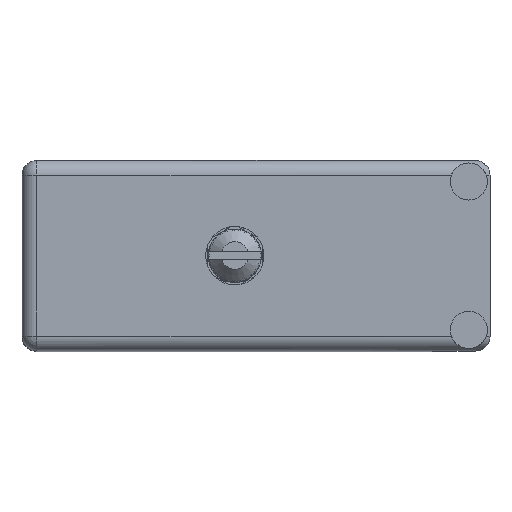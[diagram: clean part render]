
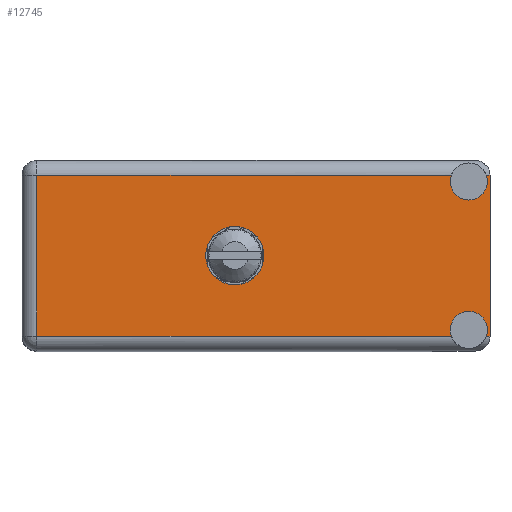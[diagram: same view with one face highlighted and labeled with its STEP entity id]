
A CAD part, top view. The second image highlights one B-rep face of the part: STEP entity #12745.
In plain terms, the highlighted face is planar.
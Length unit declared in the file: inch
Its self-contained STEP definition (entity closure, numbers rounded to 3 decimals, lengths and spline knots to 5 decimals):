
#2591 = CARTESIAN_POINT ( 'NONE',  ( 1.004, 1.566, -0.587 ) ) ;
#3348 = CARTESIAN_POINT ( 'NONE',  ( 2.208, 1.566, 0. ) ) ;
#3877 = DIRECTION ( 'NONE',  ( 0., 0., 1. ) ) ;
#5024 = ORIENTED_EDGE ( 'NONE', *, *, #66729, .F. ) ;
#6600 = EDGE_CURVE ( 'NONE', #48146, #54085, #84468, .T. ) ;
#7967 = CIRCLE ( 'NONE', #73223, 0.1375 ) ;
#8674 = VERTEX_POINT ( 'NONE', #111111 ) ;
#8995 = ORIENTED_EDGE ( 'NONE', *, *, #95544, .F. ) ;
#9302 = DIRECTION ( 'NONE',  ( 0., 1., 0. ) ) ;
#10871 = EDGE_CURVE ( 'NONE', #8674, #36048, #101424, .T. ) ;
#10915 = DIRECTION ( 'NONE',  ( 0., 1., 0. ) ) ;
#11026 = DIRECTION ( 'NONE',  ( 0., 0., 1. ) ) ;
#12745 = ADVANCED_FACE ( 'NONE', ( #70120, #63088 ), #25785, .T. ) ;
#13335 = CARTESIAN_POINT ( 'NONE',  ( 2.108, 1.566, -0.0995 ) ) ;
#14721 = CARTESIAN_POINT ( 'NONE',  ( 2.19038, 1.566, -0.829 ) ) ;
#14968 = VERTEX_POINT ( 'NONE', #64143 ) ;
#16832 = CARTESIAN_POINT ( 'NONE',  ( 2.208, 1.566, -0.07 ) ) ;
#19251 = AXIS2_PLACEMENT_3D ( 'NONE', #72174, #19673, #55251 ) ;
#19673 = DIRECTION ( 'NONE',  ( 0., 1., 0. ) ) ;
#19711 = CARTESIAN_POINT ( 'NONE',  ( 2.108, 1.566, -0.7995 ) ) ;
#20276 = ORIENTED_EDGE ( 'NONE', *, *, #80384, .F. ) ;
#20777 = CARTESIAN_POINT ( 'NONE',  ( 1.004, 1.566, -0.312 ) ) ;
#23795 = DIRECTION ( 'NONE',  ( 0., 1., 0. ) ) ;
#25191 = LINE ( 'NONE', #61328, #69030 ) ;
#25785 = PLANE ( 'NONE',  #48357 ) ;
#28217 = DIRECTION ( 'NONE',  ( 1., 0., 0. ) ) ;
#28290 = EDGE_CURVE ( 'NONE', #70112, #35660, #99480, .T. ) ;
#29414 = DIRECTION ( 'NONE',  ( -1., 0., 0. ) ) ;
#29983 = ORIENTED_EDGE ( 'NONE', *, *, #45048, .F. ) ;
#30731 = ORIENTED_EDGE ( 'NONE', *, *, #94817, .T. ) ;
#31386 = AXIS2_PLACEMENT_3D ( 'NONE', #69862, #23795, #96119 ) ;
#32620 = CARTESIAN_POINT ( 'NONE',  ( 2.208, 1.566, -0.07 ) ) ;
#32815 = EDGE_CURVE ( 'NONE', #98189, #36048, #72546, .T. ) ;
#33254 = DIRECTION ( 'NONE',  ( 0., 1., 0. ) ) ;
#35660 = VERTEX_POINT ( 'NONE', #14721 ) ;
#36048 = VERTEX_POINT ( 'NONE', #16832 ) ;
#37917 = EDGE_LOOP ( 'NONE', ( #64680, #20276, #29983, #110406, #106942, #49056, #84416, #5024, #30731, #51431 ) ) ;
#44961 = EDGE_LOOP ( 'NONE', ( #107424, #8995 ) ) ;
#45048 = EDGE_CURVE ( 'NONE', #98189, #50715, #107716, .T. ) ;
#45670 = LINE ( 'NONE', #81244, #69245 ) ;
#48146 = VERTEX_POINT ( 'NONE', #20777 ) ;
#48357 = AXIS2_PLACEMENT_3D ( 'NONE', #88787, #69545, #98694 ) ;
#48472 = CARTESIAN_POINT ( 'NONE',  ( 0.07, 1.566, -0.829 ) ) ;
#48623 = AXIS2_PLACEMENT_3D ( 'NONE', #19711, #10915, #3877 ) ;
#49056 = ORIENTED_EDGE ( 'NONE', *, *, #90664, .T. ) ;
#50715 = VERTEX_POINT ( 'NONE', #60474 ) ;
#51148 = EDGE_CURVE ( 'NONE', #55655, #14968, #25191, .T. ) ;
#51431 = ORIENTED_EDGE ( 'NONE', *, *, #51148, .T. ) ;
#53678 = CARTESIAN_POINT ( 'NONE',  ( 1.004, 1.566, -0.4495 ) ) ;
#53772 = CIRCLE ( 'NONE', #31386, 0.0875 ) ;
#54085 = VERTEX_POINT ( 'NONE', #2591 ) ;
#54191 = CIRCLE ( 'NONE', #48623, 0.0875 ) ;
#55251 = DIRECTION ( 'NONE',  ( 0., 0., 1. ) ) ;
#55655 = VERTEX_POINT ( 'NONE', #48472 ) ;
#60474 = CARTESIAN_POINT ( 'NONE',  ( 2.108, 1.566, -0.187 ) ) ;
#60769 = DIRECTION ( 'NONE',  ( 0., 0., 1. ) ) ;
#61328 = CARTESIAN_POINT ( 'NONE',  ( 0.07, 1.566, -0.899 ) ) ;
#63088 = FACE_OUTER_BOUND ( 'NONE', #37917, .T. ) ;
#64143 = CARTESIAN_POINT ( 'NONE',  ( 0.07, 1.566, -0.07 ) ) ;
#64680 = ORIENTED_EDGE ( 'NONE', *, *, #108766, .T. ) ;
#66729 = EDGE_CURVE ( 'NONE', #109293, #70112, #54191, .T. ) ;
#67032 = LINE ( 'NONE', #32620, #83664 ) ;
#67667 = CARTESIAN_POINT ( 'NONE',  ( 2.108, 1.566, -0.7995 ) ) ;
#69030 = VECTOR ( 'NONE', #60769, 39.37008 ) ;
#69245 = VECTOR ( 'NONE', #72466, 39.37008 ) ;
#69545 = DIRECTION ( 'NONE',  ( 0., 1., 0. ) ) ;
#69606 = CARTESIAN_POINT ( 'NONE',  ( 2.108, 1.566, -0.712 ) ) ;
#69862 = CARTESIAN_POINT ( 'NONE',  ( 2.108, 1.566, -0.0995 ) ) ;
#70112 = VERTEX_POINT ( 'NONE', #69606 ) ;
#70120 = FACE_BOUND ( 'NONE', #44961, .T. ) ;
#72174 = CARTESIAN_POINT ( 'NONE',  ( 1.004, 1.566, -0.4495 ) ) ;
#72403 = VECTOR ( 'NONE', #100266, 39.37008 ) ;
#72466 = DIRECTION ( 'NONE',  ( -1., 0., 0. ) ) ;
#72546 = LINE ( 'NONE', #74698, #106995 ) ;
#72921 = VERTEX_POINT ( 'NONE', #98402 ) ;
#73223 = AXIS2_PLACEMENT_3D ( 'NONE', #53678, #9302, #11026 ) ;
#74698 = CARTESIAN_POINT ( 'NONE',  ( 2.208, 1.566, -0.07 ) ) ;
#75477 = CARTESIAN_POINT ( 'NONE',  ( 0., 1.566, -0.829 ) ) ;
#76357 = DIRECTION ( 'NONE',  ( 1., 0., 0. ) ) ;
#78912 = VECTOR ( 'NONE', #29414, 39.37008 ) ;
#80384 = EDGE_CURVE ( 'NONE', #50715, #72921, #53772, .T. ) ;
#81244 = CARTESIAN_POINT ( 'NONE',  ( 0., 1.566, -0.829 ) ) ;
#82643 = AXIS2_PLACEMENT_3D ( 'NONE', #67667, #33254, #94508 ) ;
#83664 = VECTOR ( 'NONE', #76357, 39.37008 ) ;
#84416 = ORIENTED_EDGE ( 'NONE', *, *, #28290, .F. ) ;
#84468 = CIRCLE ( 'NONE', #19251, 0.1375 ) ;
#88787 = CARTESIAN_POINT ( 'NONE',  ( 0., 1.566, -0.899 ) ) ;
#90664 = EDGE_CURVE ( 'NONE', #8674, #35660, #45670, .T. ) ;
#92136 = DIRECTION ( 'NONE',  ( 0., 1., 0. ) ) ;
#94167 = CARTESIAN_POINT ( 'NONE',  ( 2.02562, 1.566, -0.829 ) ) ;
#94508 = DIRECTION ( 'NONE',  ( 0., 0., 1. ) ) ;
#94817 = EDGE_CURVE ( 'NONE', #109293, #55655, #101178, .T. ) ;
#95544 = EDGE_CURVE ( 'NONE', #54085, #48146, #7967, .T. ) ;
#96119 = DIRECTION ( 'NONE',  ( 0., 0., 1. ) ) ;
#96539 = AXIS2_PLACEMENT_3D ( 'NONE', #13335, #92136, #102065 ) ;
#98189 = VERTEX_POINT ( 'NONE', #108536 ) ;
#98402 = CARTESIAN_POINT ( 'NONE',  ( 2.02562, 1.566, -0.07 ) ) ;
#98694 = DIRECTION ( 'NONE',  ( 0., 0., 1. ) ) ;
#99480 = CIRCLE ( 'NONE', #82643, 0.0875 ) ;
#100266 = DIRECTION ( 'NONE',  ( 0., 0., 1. ) ) ;
#101178 = LINE ( 'NONE', #75477, #78912 ) ;
#101424 = LINE ( 'NONE', #3348, #72403 ) ;
#102065 = DIRECTION ( 'NONE',  ( 0., 0., 1. ) ) ;
#106942 = ORIENTED_EDGE ( 'NONE', *, *, #10871, .F. ) ;
#106995 = VECTOR ( 'NONE', #28217, 39.37008 ) ;
#107424 = ORIENTED_EDGE ( 'NONE', *, *, #6600, .F. ) ;
#107716 = CIRCLE ( 'NONE', #96539, 0.0875 ) ;
#108536 = CARTESIAN_POINT ( 'NONE',  ( 2.19038, 1.566, -0.07 ) ) ;
#108766 = EDGE_CURVE ( 'NONE', #14968, #72921, #67032, .T. ) ;
#109293 = VERTEX_POINT ( 'NONE', #94167 ) ;
#110406 = ORIENTED_EDGE ( 'NONE', *, *, #32815, .T. ) ;
#111111 = CARTESIAN_POINT ( 'NONE',  ( 2.208, 1.566, -0.829 ) ) ;
